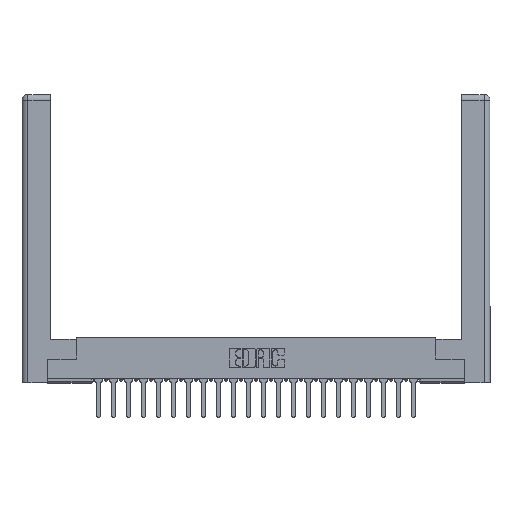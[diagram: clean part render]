
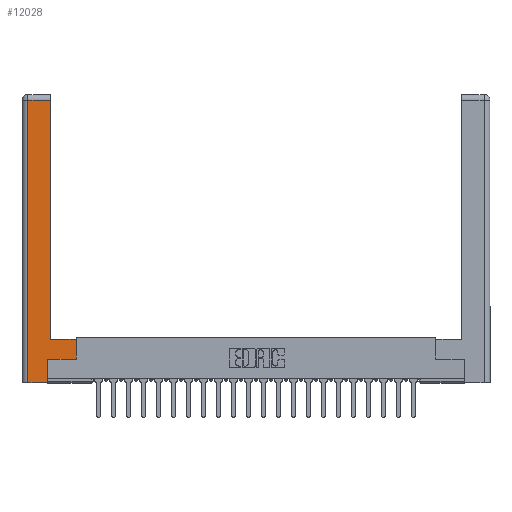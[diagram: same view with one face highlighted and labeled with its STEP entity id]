
A CAD part, top view. The second image highlights one B-rep face of the part: STEP entity #12028.
In plain terms, the highlighted planar face has unit normal (0, 0, 1).
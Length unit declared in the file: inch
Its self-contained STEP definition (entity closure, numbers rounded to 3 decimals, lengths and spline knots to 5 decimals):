
#133 = LINE ( 'NONE', #3410, #6987 ) ;
#425 = EDGE_CURVE ( 'NONE', #3855, #15283, #20556, .T. ) ;
#612 = VECTOR ( 'NONE', #5533, 39.37008 ) ;
#1136 = ORIENTED_EDGE ( 'NONE', *, *, #3719, .T. ) ;
#2832 = CARTESIAN_POINT ( 'NONE',  ( 0.295, 2.94, 0. ) ) ;
#2878 = DIRECTION ( 'NONE',  ( 0., 1., 0. ) ) ;
#3111 = CARTESIAN_POINT ( 'NONE',  ( 0.565, 0.245, 0. ) ) ;
#3410 = CARTESIAN_POINT ( 'NONE',  ( 0.0615, 0., 0. ) ) ;
#3435 = LINE ( 'NONE', #19436, #24269 ) ;
#3719 = EDGE_CURVE ( 'NONE', #5247, #3855, #16685, .T. ) ;
#3855 = VERTEX_POINT ( 'NONE', #24445 ) ;
#4081 = VERTEX_POINT ( 'NONE', #17327 ) ;
#4581 = EDGE_CURVE ( 'NONE', #15283, #4081, #19611, .T. ) ;
#5006 = LINE ( 'NONE', #8252, #20179 ) ;
#5184 = DIRECTION ( 'NONE',  ( 0., 0., -1. ) ) ;
#5192 = ORIENTED_EDGE ( 'NONE', *, *, #18912, .T. ) ;
#5246 = LINE ( 'NONE', #16731, #24013 ) ;
#5247 = VERTEX_POINT ( 'NONE', #21101 ) ;
#5533 = DIRECTION ( 'NONE',  ( 1., 0., 0. ) ) ;
#5952 = DIRECTION ( 'NONE',  ( 0., 1., 0. ) ) ;
#6825 = DIRECTION ( 'NONE',  ( -1., 0., 0. ) ) ;
#6947 = ORIENTED_EDGE ( 'NONE', *, *, #13800, .T. ) ;
#6987 = VECTOR ( 'NONE', #14664, 39.37008 ) ;
#8212 = CARTESIAN_POINT ( 'NONE',  ( 0.0615, 2.94, 0. ) ) ;
#8252 = CARTESIAN_POINT ( 'NONE',  ( 0.265, 0., 0. ) ) ;
#9102 = PLANE ( 'NONE',  #14254 ) ;
#9530 = ORIENTED_EDGE ( 'NONE', *, *, #4581, .T. ) ;
#10609 = CARTESIAN_POINT ( 'NONE',  ( 0.0615, 0., 0. ) ) ;
#10754 = EDGE_CURVE ( 'NONE', #21356, #18897, #5246, .T. ) ;
#11923 = VERTEX_POINT ( 'NONE', #10609 ) ;
#12028 = ADVANCED_FACE ( 'NONE', ( #18104 ), #9102, .F. ) ;
#12311 = CARTESIAN_POINT ( 'NONE',  ( 0.295, 0.45, 0. ) ) ;
#12748 = CARTESIAN_POINT ( 'NONE',  ( 0., 0., 0. ) ) ;
#12996 = CARTESIAN_POINT ( 'NONE',  ( 0.295, 0.45, 0. ) ) ;
#13800 = EDGE_CURVE ( 'NONE', #11923, #5247, #5006, .T. ) ;
#14066 = DIRECTION ( 'NONE',  ( 1., 0., 0. ) ) ;
#14254 = AXIS2_PLACEMENT_3D ( 'NONE', #12748, #5184, #14820 ) ;
#14664 = DIRECTION ( 'NONE',  ( 0., -1., 0. ) ) ;
#14820 = DIRECTION ( 'NONE',  ( -1., 0., 0. ) ) ;
#14944 = ORIENTED_EDGE ( 'NONE', *, *, #425, .T. ) ;
#15283 = VERTEX_POINT ( 'NONE', #21998 ) ;
#15855 = EDGE_CURVE ( 'NONE', #18897, #11923, #133, .T. ) ;
#15949 = ORIENTED_EDGE ( 'NONE', *, *, #15855, .T. ) ;
#16380 = VECTOR ( 'NONE', #2878, 39.37008 ) ;
#16685 = LINE ( 'NONE', #18352, #16380 ) ;
#16731 = CARTESIAN_POINT ( 'NONE',  ( 0.0615, 2.94, 0. ) ) ;
#17069 = VECTOR ( 'NONE', #6825, 39.37008 ) ;
#17327 = CARTESIAN_POINT ( 'NONE',  ( 0.565, 0.45, 0. ) ) ;
#18104 = FACE_OUTER_BOUND ( 'NONE', #23527, .T. ) ;
#18352 = CARTESIAN_POINT ( 'NONE',  ( 0.265, 0.245, 0. ) ) ;
#18881 = LINE ( 'NONE', #12311, #17069 ) ;
#18897 = VERTEX_POINT ( 'NONE', #8212 ) ;
#18912 = EDGE_CURVE ( 'NONE', #23792, #21356, #3435, .T. ) ;
#19436 = CARTESIAN_POINT ( 'NONE',  ( 0.295, 3., 0. ) ) ;
#19611 = LINE ( 'NONE', #23097, #23215 ) ;
#19694 = EDGE_CURVE ( 'NONE', #4081, #23792, #18881, .T. ) ;
#19798 = ORIENTED_EDGE ( 'NONE', *, *, #19694, .T. ) ;
#20179 = VECTOR ( 'NONE', #14066, 39.37008 ) ;
#20556 = LINE ( 'NONE', #3111, #612 ) ;
#21101 = CARTESIAN_POINT ( 'NONE',  ( 0.265, 0., 0. ) ) ;
#21334 = DIRECTION ( 'NONE',  ( 0., 1., 0. ) ) ;
#21356 = VERTEX_POINT ( 'NONE', #2832 ) ;
#21998 = CARTESIAN_POINT ( 'NONE',  ( 0.565, 0.245, 0. ) ) ;
#22653 = DIRECTION ( 'NONE',  ( -1., 0., 0. ) ) ;
#22972 = ORIENTED_EDGE ( 'NONE', *, *, #10754, .T. ) ;
#23097 = CARTESIAN_POINT ( 'NONE',  ( 0.565, 0.45, 0. ) ) ;
#23215 = VECTOR ( 'NONE', #5952, 39.37008 ) ;
#23527 = EDGE_LOOP ( 'NONE', ( #5192, #22972, #15949, #6947, #1136, #14944, #9530, #19798 ) ) ;
#23792 = VERTEX_POINT ( 'NONE', #12996 ) ;
#24013 = VECTOR ( 'NONE', #22653, 39.37008 ) ;
#24269 = VECTOR ( 'NONE', #21334, 39.37008 ) ;
#24445 = CARTESIAN_POINT ( 'NONE',  ( 0.265, 0.245, 0. ) ) ;
